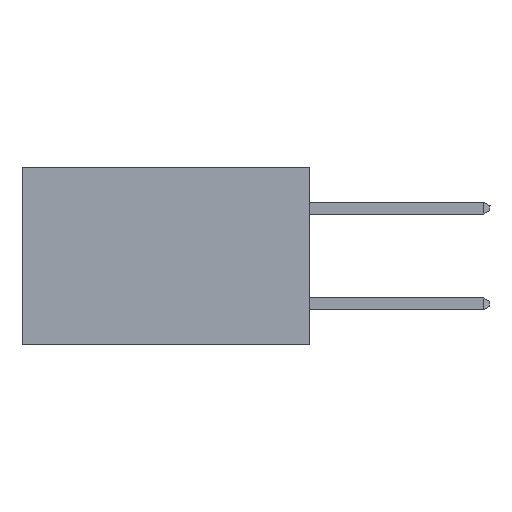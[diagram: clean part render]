
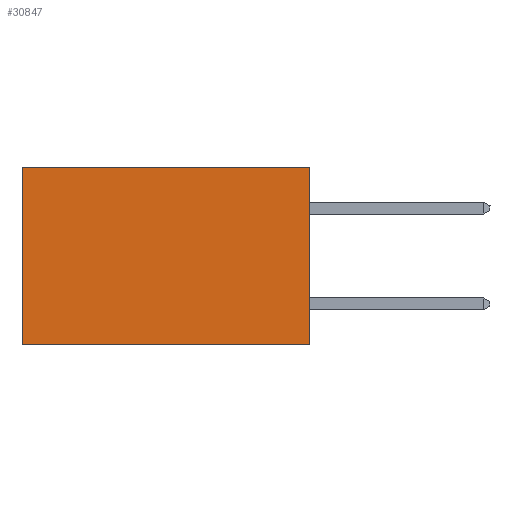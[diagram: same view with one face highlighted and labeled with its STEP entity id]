
A CAD part, left-side view. The second image highlights one B-rep face of the part: STEP entity #30847.
In plain terms, the highlighted planar face has unit normal (-1, 0, 0).
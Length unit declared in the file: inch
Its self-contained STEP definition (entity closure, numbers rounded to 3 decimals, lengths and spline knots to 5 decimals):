
#1043 = CARTESIAN_POINT ( 'NONE',  ( 0.2875, 0., -0.37 ) ) ;
#1806 = DIRECTION ( 'NONE',  ( 0., 0., -1. ) ) ;
#1925 = CARTESIAN_POINT ( 'NONE',  ( 0.2875, 0., 0. ) ) ;
#4140 = VERTEX_POINT ( 'NONE', #27652 ) ;
#5724 = DIRECTION ( 'NONE',  ( 0., 0., -1. ) ) ;
#7464 = VECTOR ( 'NONE', #22353, 39.37008 ) ;
#7865 = EDGE_CURVE ( 'NONE', #29959, #29032, #22731, .T. ) ;
#8594 = ORIENTED_EDGE ( 'NONE', *, *, #7865, .F. ) ;
#9517 = LINE ( 'NONE', #30059, #7464 ) ;
#9611 = CARTESIAN_POINT ( 'NONE',  ( 0.2875, 0.6, -0.37 ) ) ;
#9751 = VECTOR ( 'NONE', #33009, 39.37008 ) ;
#10495 = EDGE_CURVE ( 'NONE', #29648, #29959, #9517, .T. ) ;
#10856 = ORIENTED_EDGE ( 'NONE', *, *, #33167, .T. ) ;
#12020 = PLANE ( 'NONE',  #31926 ) ;
#13987 = DIRECTION ( 'NONE',  ( 0., 1., 0. ) ) ;
#21135 = LINE ( 'NONE', #23935, #21955 ) ;
#21157 = LINE ( 'NONE', #22051, #9751 ) ;
#21619 = EDGE_LOOP ( 'NONE', ( #33978, #8594, #28967, #10856 ) ) ;
#21955 = VECTOR ( 'NONE', #5724, 39.37008 ) ;
#22051 = CARTESIAN_POINT ( 'NONE',  ( 0.2875, 0., 0. ) ) ;
#22353 = DIRECTION ( 'NONE',  ( 0., 0., -1. ) ) ;
#22731 = LINE ( 'NONE', #1043, #24763 ) ;
#22878 = DIRECTION ( 'NONE',  ( 1., 0., 0. ) ) ;
#23935 = CARTESIAN_POINT ( 'NONE',  ( 0.2875, 0.6, 0. ) ) ;
#24763 = VECTOR ( 'NONE', #13987, 39.37008 ) ;
#26255 = CARTESIAN_POINT ( 'NONE',  ( 0.2875, 0., 0. ) ) ;
#27652 = CARTESIAN_POINT ( 'NONE',  ( 0.2875, 0.6, 0. ) ) ;
#28360 = EDGE_CURVE ( 'NONE', #4140, #29032, #21135, .T. ) ;
#28967 = ORIENTED_EDGE ( 'NONE', *, *, #10495, .F. ) ;
#29032 = VERTEX_POINT ( 'NONE', #9611 ) ;
#29193 = FACE_OUTER_BOUND ( 'NONE', #21619, .T. ) ;
#29648 = VERTEX_POINT ( 'NONE', #26255 ) ;
#29959 = VERTEX_POINT ( 'NONE', #32582 ) ;
#30059 = CARTESIAN_POINT ( 'NONE',  ( 0.2875, 0., 0. ) ) ;
#30847 = ADVANCED_FACE ( 'NONE', ( #29193 ), #12020, .F. ) ;
#31926 = AXIS2_PLACEMENT_3D ( 'NONE', #1925, #22878, #1806 ) ;
#32582 = CARTESIAN_POINT ( 'NONE',  ( 0.2875, 0., -0.37 ) ) ;
#33009 = DIRECTION ( 'NONE',  ( 0., 1., 0. ) ) ;
#33167 = EDGE_CURVE ( 'NONE', #29648, #4140, #21157, .T. ) ;
#33978 = ORIENTED_EDGE ( 'NONE', *, *, #28360, .T. ) ;
